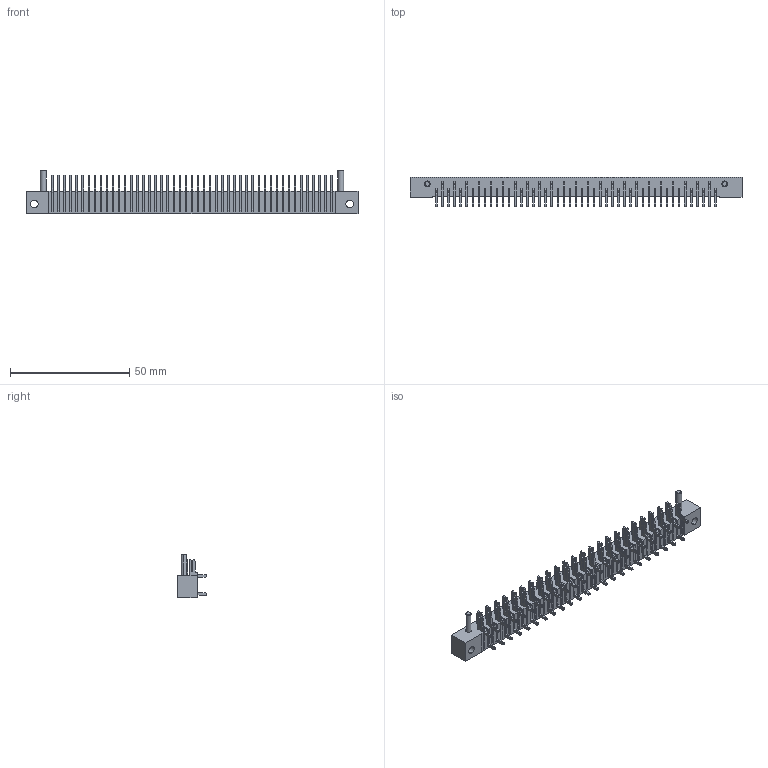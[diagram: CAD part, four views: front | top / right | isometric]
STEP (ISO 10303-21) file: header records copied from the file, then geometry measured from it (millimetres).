
FILE_DESCRIPTION (( 'STEP AP203' ), '1' );
FILE_NAME ('423-047-521-102.STEP', '2019-11-28T19:50:29', ( '' ), ( '' ), 'SwSTEP 2.0', 'SolidWorks 2016', '' );
FILE_SCHEMA (( 'CONFIG_CONTROL_DESIGN' ));
Length unit declared in the file: inch
Products named in the file (4): 421-290-001_121; 421-290-002_121; 423 Part_47; 423-047-521-102
Assembly tree (48 placements, depth 2):
  423-047-521-102
    423 Part_47
    421-290-001_121  x23
    421-290-002_121  x24
Bounding box: 138.94 x 12.19 x 18.29 mm (x, y, z)
Volume: 10689.3 mm3; surface area: 16426.6 mm2
Topology: 48 solids, 48 shells, 1573 faces, 4396 edges, 2928 vertices
Faces by surface type: plane 1283, cylinder 286, cone 4
Entity records: 13356 total; most frequent: CARTESIAN_POINT 2114, ORIENTED_EDGE 2036, DIRECTION 1948, EDGE_CURVE 1018, VECTOR 896, LINE 896, VERTEX_POINT 676, AXIS2_PLACEMENT_3D 526
